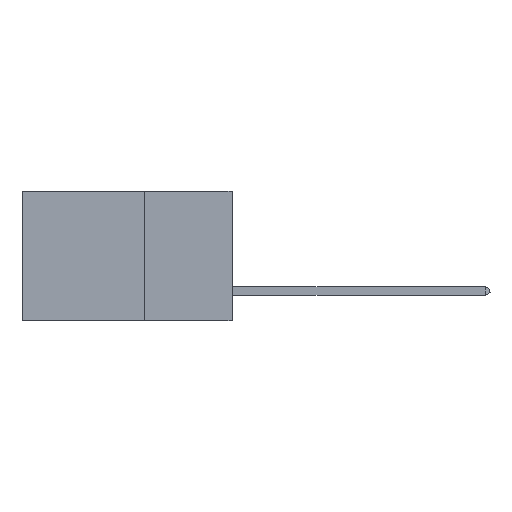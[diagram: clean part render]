
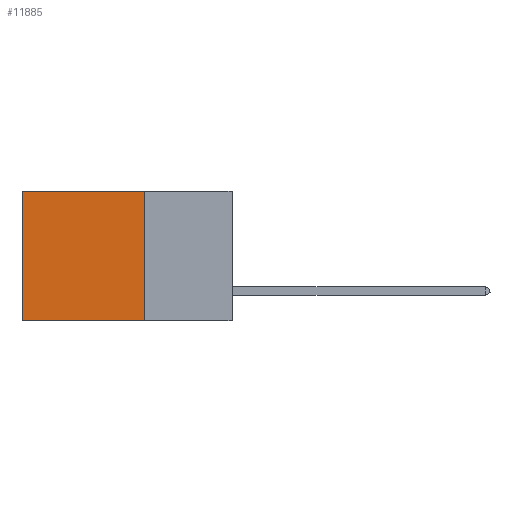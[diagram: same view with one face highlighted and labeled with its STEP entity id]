
A CAD part, left-side view. The second image highlights one B-rep face of the part: STEP entity #11885.
In plain terms, the highlighted planar face has unit normal (-1, 0, 0).
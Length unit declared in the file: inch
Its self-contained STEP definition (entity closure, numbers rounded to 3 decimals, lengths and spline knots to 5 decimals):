
#164 = PLANE ( 'NONE',  #2153 ) ;
#760 = ORIENTED_EDGE ( 'NONE', *, *, #13244, .T. ) ;
#1030 = EDGE_CURVE ( 'NONE', #12487, #10478, #12512, .T. ) ;
#2002 = EDGE_LOOP ( 'NONE', ( #2870, #6539, #9864, #760 ) ) ;
#2047 = CARTESIAN_POINT ( 'NONE',  ( 0.2875, 0.25, 0. ) ) ;
#2153 = AXIS2_PLACEMENT_3D ( 'NONE', #10216, #11641, #3048 ) ;
#2637 = LINE ( 'NONE', #10786, #3331 ) ;
#2870 = ORIENTED_EDGE ( 'NONE', *, *, #13490, .T. ) ;
#2957 = CARTESIAN_POINT ( 'NONE',  ( 0.2875, 0.6, 0. ) ) ;
#2999 = EDGE_CURVE ( 'NONE', #10478, #17602, #12646, .T. ) ;
#3025 = DIRECTION ( 'NONE',  ( 0., 1., 0. ) ) ;
#3048 = DIRECTION ( 'NONE',  ( 0., 0., -1. ) ) ;
#3331 = VECTOR ( 'NONE', #12252, 39.37008 ) ;
#6539 = ORIENTED_EDGE ( 'NONE', *, *, #2999, .F. ) ;
#7424 = DIRECTION ( 'NONE',  ( 0., 0., -1. ) ) ;
#7775 = CARTESIAN_POINT ( 'NONE',  ( 0.2875, 0.25, 0. ) ) ;
#8165 = CARTESIAN_POINT ( 'NONE',  ( 0.2875, 0.25, -0.37 ) ) ;
#9849 = CARTESIAN_POINT ( 'NONE',  ( 0.2875, 0.6, 0. ) ) ;
#9864 = ORIENTED_EDGE ( 'NONE', *, *, #1030, .F. ) ;
#10216 = CARTESIAN_POINT ( 'NONE',  ( 0.2875, 0.25, 0. ) ) ;
#10478 = VERTEX_POINT ( 'NONE', #8165 ) ;
#10508 = VECTOR ( 'NONE', #7424, 39.37008 ) ;
#10786 = CARTESIAN_POINT ( 'NONE',  ( 0.2875, 0.25, 0. ) ) ;
#11036 = FACE_OUTER_BOUND ( 'NONE', #2002, .T. ) ;
#11127 = VECTOR ( 'NONE', #15093, 39.37008 ) ;
#11641 = DIRECTION ( 'NONE',  ( 1., 0., 0. ) ) ;
#11885 = ADVANCED_FACE ( 'NONE', ( #11036 ), #164, .F. ) ;
#12252 = DIRECTION ( 'NONE',  ( 0., 1., 0. ) ) ;
#12487 = VERTEX_POINT ( 'NONE', #7775 ) ;
#12512 = LINE ( 'NONE', #2047, #11127 ) ;
#12646 = LINE ( 'NONE', #14739, #15143 ) ;
#13244 = EDGE_CURVE ( 'NONE', #12487, #13268, #2637, .T. ) ;
#13268 = VERTEX_POINT ( 'NONE', #9849 ) ;
#13490 = EDGE_CURVE ( 'NONE', #13268, #17602, #14791, .T. ) ;
#14739 = CARTESIAN_POINT ( 'NONE',  ( 0.2875, 0.25, -0.37 ) ) ;
#14791 = LINE ( 'NONE', #2957, #10508 ) ;
#15093 = DIRECTION ( 'NONE',  ( 0., 0., -1. ) ) ;
#15143 = VECTOR ( 'NONE', #3025, 39.37008 ) ;
#15282 = CARTESIAN_POINT ( 'NONE',  ( 0.2875, 0.6, -0.37 ) ) ;
#17602 = VERTEX_POINT ( 'NONE', #15282 ) ;
